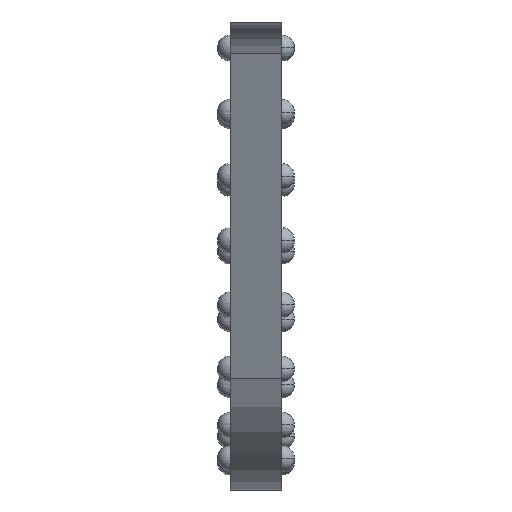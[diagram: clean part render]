
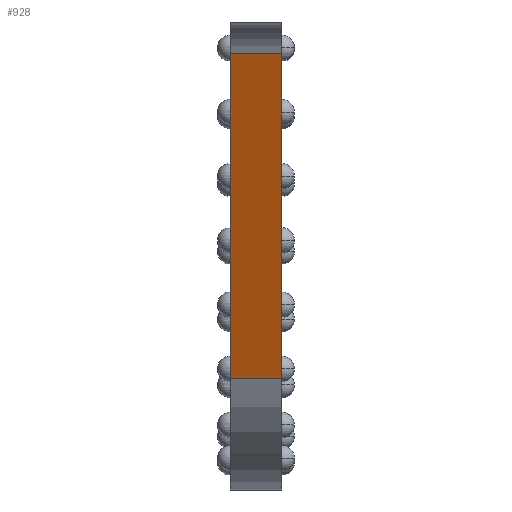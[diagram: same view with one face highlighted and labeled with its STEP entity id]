
A CAD part, top view. The second image highlights one B-rep face of the part: STEP entity #928.
In plain terms, the highlighted planar face has unit normal (0, -0.383, 0.924).
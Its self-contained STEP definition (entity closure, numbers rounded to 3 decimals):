
#18 = LINE ( 'NONE', #1456, #1839 ) ;
#34 = VERTEX_POINT ( 'NONE', #598 ) ;
#172 = DIRECTION ( 'NONE',  ( 0., 0.383, -0.924 ) ) ;
#205 = VECTOR ( 'NONE', #1440, 1000. ) ;
#375 = VERTEX_POINT ( 'NONE', #841 ) ;
#386 = VECTOR ( 'NONE', #1462, 1000. ) ;
#403 = ORIENTED_EDGE ( 'NONE', *, *, #1280, .F. ) ;
#441 = CARTESIAN_POINT ( 'NONE',  ( 0., -61.173, -11.79 ) ) ;
#443 = CARTESIAN_POINT ( 'NONE',  ( 0., -4.79, 11.565 ) ) ;
#469 = CARTESIAN_POINT ( 'NONE',  ( 0., -124.291, -37.934 ) ) ;
#598 = CARTESIAN_POINT ( 'NONE',  ( 0., -61.173, -11.79 ) ) ;
#599 = LINE ( 'NONE', #728, #205 ) ;
#608 = DIRECTION ( 'NONE',  ( -1., 0., 0. ) ) ;
#728 = CARTESIAN_POINT ( 'NONE',  ( 10., -4.79, 11.565 ) ) ;
#776 = EDGE_CURVE ( 'NONE', #375, #34, #1244, .T. ) ;
#841 = CARTESIAN_POINT ( 'NONE',  ( 10., -61.173, -11.79 ) ) ;
#862 = ORIENTED_EDGE ( 'NONE', *, *, #1449, .F. ) ;
#891 = ORIENTED_EDGE ( 'NONE', *, *, #776, .T. ) ;
#898 = DIRECTION ( 'NONE',  ( -1., 0., 0. ) ) ;
#928 = ADVANCED_FACE ( 'NONE', ( #1398 ), #1065, .F. ) ;
#1042 = EDGE_LOOP ( 'NONE', ( #403, #891, #1446, #862 ) ) ;
#1065 = PLANE ( 'NONE',  #1283 ) ;
#1193 = VECTOR ( 'NONE', #608, 1000. ) ;
#1211 = DIRECTION ( 'NONE',  ( 0., 0.924, 0.383 ) ) ;
#1244 = LINE ( 'NONE', #441, #1193 ) ;
#1247 = CARTESIAN_POINT ( 'NONE',  ( 10., -124.291, -37.934 ) ) ;
#1280 = EDGE_CURVE ( 'NONE', #375, #1780, #599, .T. ) ;
#1283 = AXIS2_PLACEMENT_3D ( 'NONE', #1757, #172, #1211 ) ;
#1398 = FACE_OUTER_BOUND ( 'NONE', #1042, .T. ) ;
#1440 = DIRECTION ( 'NONE',  ( 0., -0.924, -0.383 ) ) ;
#1446 = ORIENTED_EDGE ( 'NONE', *, *, #1564, .T. ) ;
#1449 = EDGE_CURVE ( 'NONE', #1780, #1642, #18, .T. ) ;
#1456 = CARTESIAN_POINT ( 'NONE',  ( 10., -124.291, -37.934 ) ) ;
#1462 = DIRECTION ( 'NONE',  ( 0., -0.924, -0.383 ) ) ;
#1502 = LINE ( 'NONE', #443, #386 ) ;
#1564 = EDGE_CURVE ( 'NONE', #34, #1642, #1502, .T. ) ;
#1642 = VERTEX_POINT ( 'NONE', #469 ) ;
#1757 = CARTESIAN_POINT ( 'NONE',  ( 10., -4.79, 11.565 ) ) ;
#1780 = VERTEX_POINT ( 'NONE', #1247 ) ;
#1839 = VECTOR ( 'NONE', #898, 1000. ) ;
